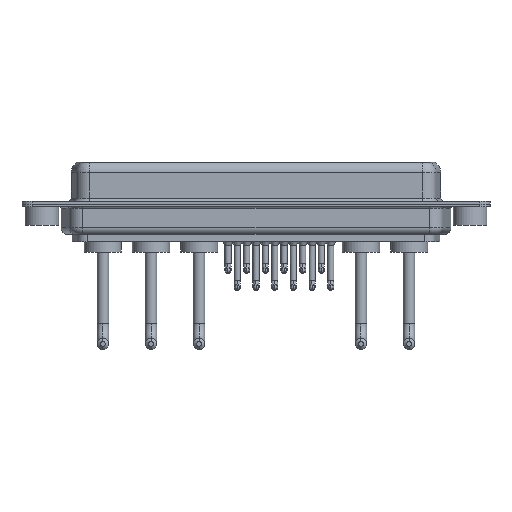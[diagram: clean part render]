
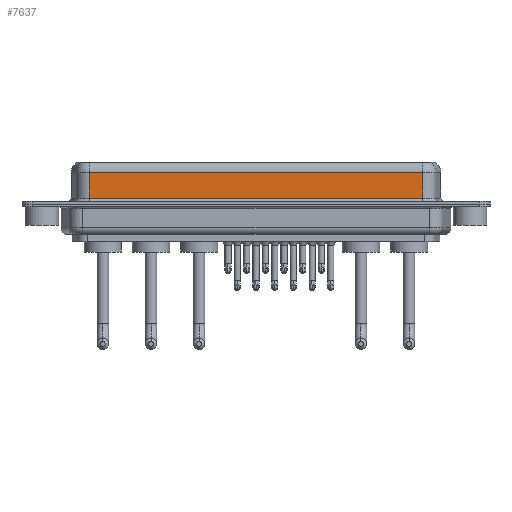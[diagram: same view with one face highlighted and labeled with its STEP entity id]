
A CAD part, front view. The second image highlights one B-rep face of the part: STEP entity #7637.
In plain terms, the highlighted planar face has unit normal (0, -1, 0).
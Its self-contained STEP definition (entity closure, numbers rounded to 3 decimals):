
#246 = CARTESIAN_POINT ( 'NONE',  ( 7.038, -3.95, 4.65 ) ) ;
#632 = LINE ( 'NONE', #3490, #8141 ) ;
#2088 = LINE ( 'NONE', #8250, #9392 ) ;
#2538 = AXIS2_PLACEMENT_3D ( 'NONE', #14087, #12235, #18727 ) ;
#3034 = CARTESIAN_POINT ( 'NONE',  ( 56.462, -3.95, 4.65 ) ) ;
#3490 = CARTESIAN_POINT ( 'NONE',  ( 56.462, -3.95, 0.9 ) ) ;
#5201 = ORIENTED_EDGE ( 'NONE', *, *, #19683, .T. ) ;
#5552 = CARTESIAN_POINT ( 'NONE',  ( 7.038, -3.95, 6.4 ) ) ;
#7637 = ADVANCED_FACE ( 'NONE', ( #11630 ), #17913, .F. ) ;
#8141 = VECTOR ( 'NONE', #14546, 1000. ) ;
#8193 = EDGE_CURVE ( 'NONE', #14411, #19615, #632, .T. ) ;
#8250 = CARTESIAN_POINT ( 'NONE',  ( 56.462, -3.95, 4.65 ) ) ;
#8388 = EDGE_CURVE ( 'NONE', #16811, #14411, #18352, .T. ) ;
#9392 = VECTOR ( 'NONE', #19226, 1000. ) ;
#9942 = CARTESIAN_POINT ( 'NONE',  ( 56.462, -3.95, 6.4 ) ) ;
#10054 = ORIENTED_EDGE ( 'NONE', *, *, #8388, .T. ) ;
#11630 = FACE_OUTER_BOUND ( 'NONE', #12617, .T. ) ;
#11677 = EDGE_CURVE ( 'NONE', #12360, #19615, #17756, .T. ) ;
#12235 = DIRECTION ( 'NONE',  ( 0., 1., 0. ) ) ;
#12360 = VERTEX_POINT ( 'NONE', #3034 ) ;
#12617 = EDGE_LOOP ( 'NONE', ( #15399, #5201, #10054, #19735 ) ) ;
#14087 = CARTESIAN_POINT ( 'NONE',  ( 56.462, -3.95, 6.4 ) ) ;
#14411 = VERTEX_POINT ( 'NONE', #14958 ) ;
#14546 = DIRECTION ( 'NONE',  ( 1., 0., 0. ) ) ;
#14958 = CARTESIAN_POINT ( 'NONE',  ( 7.038, -3.95, 0.9 ) ) ;
#15399 = ORIENTED_EDGE ( 'NONE', *, *, #11677, .F. ) ;
#16121 = CARTESIAN_POINT ( 'NONE',  ( 56.462, -3.95, 0.9 ) ) ;
#16202 = DIRECTION ( 'NONE',  ( 0., 0., -1. ) ) ;
#16811 = VERTEX_POINT ( 'NONE', #246 ) ;
#16899 = DIRECTION ( 'NONE',  ( 0., 0., -1. ) ) ;
#17756 = LINE ( 'NONE', #9942, #19699 ) ;
#17913 = PLANE ( 'NONE',  #2538 ) ;
#18299 = VECTOR ( 'NONE', #16899, 1000. ) ;
#18352 = LINE ( 'NONE', #5552, #18299 ) ;
#18727 = DIRECTION ( 'NONE',  ( 0., 0., 1. ) ) ;
#19226 = DIRECTION ( 'NONE',  ( -1., 0., 0. ) ) ;
#19615 = VERTEX_POINT ( 'NONE', #16121 ) ;
#19683 = EDGE_CURVE ( 'NONE', #12360, #16811, #2088, .T. ) ;
#19699 = VECTOR ( 'NONE', #16202, 1000. ) ;
#19735 = ORIENTED_EDGE ( 'NONE', *, *, #8193, .T. ) ;
